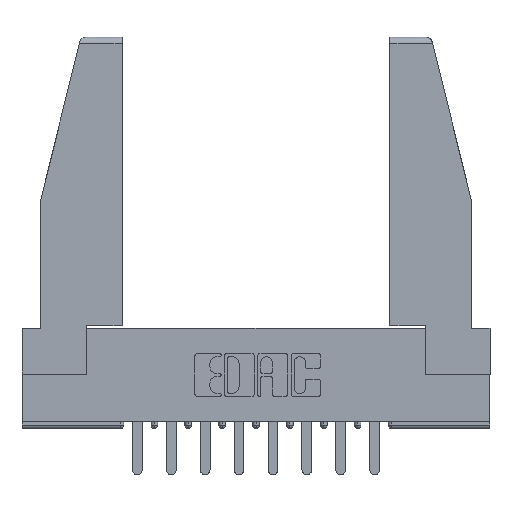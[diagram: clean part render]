
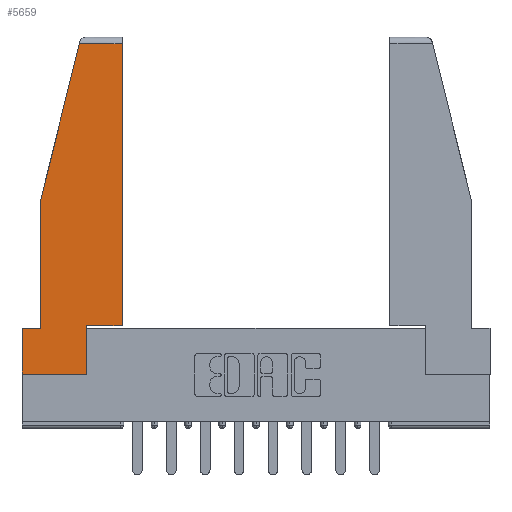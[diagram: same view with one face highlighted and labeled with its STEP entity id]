
A CAD part, top view. The second image highlights one B-rep face of the part: STEP entity #5659.
In plain terms, the highlighted planar face has unit normal (0, 0, 1).
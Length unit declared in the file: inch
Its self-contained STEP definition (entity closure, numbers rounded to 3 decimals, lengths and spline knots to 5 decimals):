
#63 = DIRECTION ( 'NONE',  ( 0., -1., 0. ) ) ;
#170 = EDGE_CURVE ( 'NONE', #2721, #14041, #14107, .T. ) ;
#306 = VERTEX_POINT ( 'NONE', #6740 ) ;
#372 = VECTOR ( 'NONE', #63, 39.37008 ) ;
#537 = CARTESIAN_POINT ( 'NONE',  ( 0., 0., 0. ) ) ;
#648 = EDGE_CURVE ( 'NONE', #14135, #14744, #4972, .T. ) ;
#664 = CARTESIAN_POINT ( 'NONE',  ( 0.271, 1.55, 0. ) ) ;
#799 = VECTOR ( 'NONE', #13933, 39.37008 ) ;
#867 = EDGE_CURVE ( 'NONE', #8293, #13643, #1819, .T. ) ;
#998 = VECTOR ( 'NONE', #1223, 39.37008 ) ;
#1194 = CARTESIAN_POINT ( 'NONE',  ( 0., 0.21, 0. ) ) ;
#1223 = DIRECTION ( 'NONE',  ( 1., 0., 0. ) ) ;
#1350 = EDGE_CURVE ( 'NONE', #13643, #306, #12090, .T. ) ;
#1819 = LINE ( 'NONE', #4625, #3673 ) ;
#2260 = CARTESIAN_POINT ( 'NONE',  ( 0., 0., 0. ) ) ;
#2530 = CARTESIAN_POINT ( 'NONE',  ( 0., 0.21, 0. ) ) ;
#2721 = VERTEX_POINT ( 'NONE', #9721 ) ;
#2759 = DIRECTION ( 'NONE',  ( 0., 0., 1. ) ) ;
#3087 = ORIENTED_EDGE ( 'NONE', *, *, #7433, .T. ) ;
#3175 = VECTOR ( 'NONE', #9431, 39.37008 ) ;
#3673 = VECTOR ( 'NONE', #12944, 39.37008 ) ;
#4241 = DIRECTION ( 'NONE',  ( 0., -1., 0. ) ) ;
#4625 = CARTESIAN_POINT ( 'NONE',  ( 0.461, 0.223, 0. ) ) ;
#4810 = CARTESIAN_POINT ( 'NONE',  ( 0., 1.52, 0. ) ) ;
#4972 = LINE ( 'NONE', #2530, #372 ) ;
#5383 = DIRECTION ( 'NONE',  ( -0.239, -0.971, 0. ) ) ;
#5472 = CARTESIAN_POINT ( 'NONE',  ( 0.086, 0.21, 0. ) ) ;
#5490 = VECTOR ( 'NONE', #14000, 39.37008 ) ;
#5598 = FACE_OUTER_BOUND ( 'NONE', #12313, .T. ) ;
#5659 = ADVANCED_FACE ( 'NONE', ( #5598 ), #11859, .T. ) ;
#5929 = ORIENTED_EDGE ( 'NONE', *, *, #9882, .T. ) ;
#6348 = ORIENTED_EDGE ( 'NONE', *, *, #8936, .T. ) ;
#6660 = ORIENTED_EDGE ( 'NONE', *, *, #648, .T. ) ;
#6740 = CARTESIAN_POINT ( 'NONE',  ( 0.2636, 1.52, 0. ) ) ;
#6985 = VECTOR ( 'NONE', #4241, 39.37008 ) ;
#7117 = ORIENTED_EDGE ( 'NONE', *, *, #14309, .T. ) ;
#7433 = EDGE_CURVE ( 'NONE', #13507, #14131, #11777, .T. ) ;
#7580 = VECTOR ( 'NONE', #5383, 39.37008 ) ;
#8293 = VERTEX_POINT ( 'NONE', #8433 ) ;
#8433 = CARTESIAN_POINT ( 'NONE',  ( 0.461, 0.223, 0. ) ) ;
#8541 = ORIENTED_EDGE ( 'NONE', *, *, #1350, .T. ) ;
#8684 = CARTESIAN_POINT ( 'NONE',  ( 0.297, 0., 0. ) ) ;
#8936 = EDGE_CURVE ( 'NONE', #14744, #13507, #13278, .T. ) ;
#9364 = CARTESIAN_POINT ( 'NONE',  ( 0.297, 0.223, 0. ) ) ;
#9431 = DIRECTION ( 'NONE',  ( -1., 0., 0. ) ) ;
#9587 = VECTOR ( 'NONE', #10604, 39.37008 ) ;
#9721 = CARTESIAN_POINT ( 'NONE',  ( 0.086, 0.8, 0. ) ) ;
#9882 = EDGE_CURVE ( 'NONE', #14041, #14135, #12667, .T. ) ;
#9902 = EDGE_CURVE ( 'NONE', #306, #2721, #14665, .T. ) ;
#9987 = ORIENTED_EDGE ( 'NONE', *, *, #170, .T. ) ;
#10107 = CARTESIAN_POINT ( 'NONE',  ( 0.086, 0.8, 0. ) ) ;
#10219 = CARTESIAN_POINT ( 'NONE',  ( 0., 0., 0. ) ) ;
#10604 = DIRECTION ( 'NONE',  ( 0., 1., 0. ) ) ;
#11331 = ORIENTED_EDGE ( 'NONE', *, *, #867, .T. ) ;
#11777 = LINE ( 'NONE', #12581, #9587 ) ;
#11859 = PLANE ( 'NONE',  #11905 ) ;
#11905 = AXIS2_PLACEMENT_3D ( 'NONE', #537, #2759, #12068 ) ;
#12068 = DIRECTION ( 'NONE',  ( 1., 0., 0. ) ) ;
#12090 = LINE ( 'NONE', #4810, #5490 ) ;
#12313 = EDGE_LOOP ( 'NONE', ( #11331, #8541, #13399, #9987, #5929, #6660, #6348, #3087, #7117 ) ) ;
#12373 = CARTESIAN_POINT ( 'NONE',  ( 0.297, 0.223, 0. ) ) ;
#12429 = CARTESIAN_POINT ( 'NONE',  ( 0., 0.21, 0. ) ) ;
#12581 = CARTESIAN_POINT ( 'NONE',  ( 0.297, 0., 0. ) ) ;
#12667 = LINE ( 'NONE', #1194, #3175 ) ;
#12944 = DIRECTION ( 'NONE',  ( 0., 1., 0. ) ) ;
#12975 = LINE ( 'NONE', #9364, #998 ) ;
#13278 = LINE ( 'NONE', #2260, #799 ) ;
#13399 = ORIENTED_EDGE ( 'NONE', *, *, #9902, .T. ) ;
#13507 = VERTEX_POINT ( 'NONE', #8684 ) ;
#13643 = VERTEX_POINT ( 'NONE', #13800 ) ;
#13800 = CARTESIAN_POINT ( 'NONE',  ( 0.461, 1.52, 0. ) ) ;
#13933 = DIRECTION ( 'NONE',  ( 1., 0., 0. ) ) ;
#14000 = DIRECTION ( 'NONE',  ( -1., 0., 0. ) ) ;
#14041 = VERTEX_POINT ( 'NONE', #5472 ) ;
#14107 = LINE ( 'NONE', #10107, #6985 ) ;
#14131 = VERTEX_POINT ( 'NONE', #12373 ) ;
#14135 = VERTEX_POINT ( 'NONE', #12429 ) ;
#14309 = EDGE_CURVE ( 'NONE', #14131, #8293, #12975, .T. ) ;
#14665 = LINE ( 'NONE', #664, #7580 ) ;
#14744 = VERTEX_POINT ( 'NONE', #10219 ) ;
